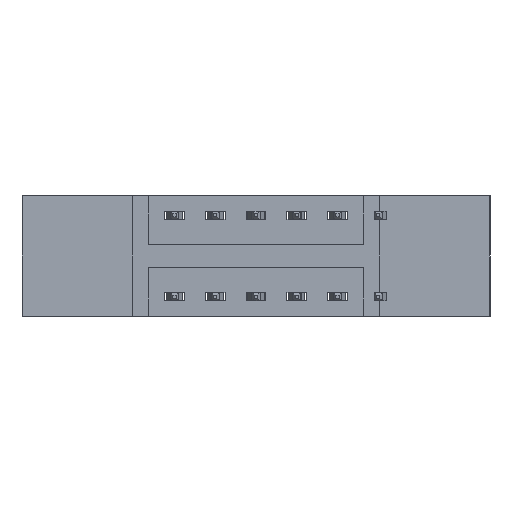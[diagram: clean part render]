
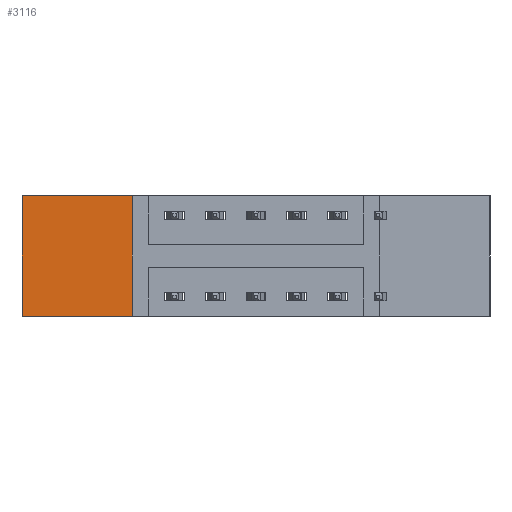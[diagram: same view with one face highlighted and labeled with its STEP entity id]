
A CAD part, front view. The second image highlights one B-rep face of the part: STEP entity #3116.
In plain terms, the highlighted planar face has unit normal (0, -1, 0).
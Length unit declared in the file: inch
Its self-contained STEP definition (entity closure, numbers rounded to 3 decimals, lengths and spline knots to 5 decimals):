
#100 = CARTESIAN_POINT ( 'NONE',  ( 0., 0.17, -0.37 ) ) ;
#230 = DIRECTION ( 'NONE',  ( 0., 0., 1. ) ) ;
#784 = DIRECTION ( 'NONE',  ( 1., 0., 0. ) ) ;
#1079 = EDGE_CURVE ( 'NONE', #4943, #7428, #5833, .T. ) ;
#1197 = CARTESIAN_POINT ( 'NONE',  ( 0.3375, 0.17, -0.37 ) ) ;
#1203 = CARTESIAN_POINT ( 'NONE',  ( 0.3375, 0.17, 0. ) ) ;
#1258 = CARTESIAN_POINT ( 'NONE',  ( 0., 0.17, 0. ) ) ;
#1836 = EDGE_CURVE ( 'NONE', #3618, #4943, #2764, .T. ) ;
#1899 = DIRECTION ( 'NONE',  ( -1., 0., 0. ) ) ;
#2666 = AXIS2_PLACEMENT_3D ( 'NONE', #4373, #3694, #6317 ) ;
#2764 = LINE ( 'NONE', #8026, #3585 ) ;
#2996 = FACE_OUTER_BOUND ( 'NONE', #7857, .T. ) ;
#3029 = ORIENTED_EDGE ( 'NONE', *, *, #1079, .T. ) ;
#3116 = ADVANCED_FACE ( 'NONE', ( #2996 ), #8420, .T. ) ;
#3242 = VECTOR ( 'NONE', #1899, 39.37008 ) ;
#3372 = LINE ( 'NONE', #4587, #5441 ) ;
#3415 = DIRECTION ( 'NONE',  ( 0., 0., -1. ) ) ;
#3585 = VECTOR ( 'NONE', #230, 39.37008 ) ;
#3618 = VERTEX_POINT ( 'NONE', #1197 ) ;
#3694 = DIRECTION ( 'NONE',  ( 0., -1., 0. ) ) ;
#4373 = CARTESIAN_POINT ( 'NONE',  ( 0., 0.17, -0.37 ) ) ;
#4587 = CARTESIAN_POINT ( 'NONE',  ( 0., 0.17, 0. ) ) ;
#4729 = EDGE_CURVE ( 'NONE', #7428, #5667, #3372, .T. ) ;
#4943 = VERTEX_POINT ( 'NONE', #1203 ) ;
#5441 = VECTOR ( 'NONE', #3415, 39.37008 ) ;
#5667 = VERTEX_POINT ( 'NONE', #6264 ) ;
#5815 = ORIENTED_EDGE ( 'NONE', *, *, #7746, .T. ) ;
#5833 = LINE ( 'NONE', #1258, #3242 ) ;
#5959 = LINE ( 'NONE', #100, #6807 ) ;
#5965 = ORIENTED_EDGE ( 'NONE', *, *, #1836, .T. ) ;
#6264 = CARTESIAN_POINT ( 'NONE',  ( 0., 0.17, -0.37 ) ) ;
#6294 = ORIENTED_EDGE ( 'NONE', *, *, #4729, .T. ) ;
#6317 = DIRECTION ( 'NONE',  ( 0., 0., -1. ) ) ;
#6807 = VECTOR ( 'NONE', #784, 39.37008 ) ;
#7428 = VERTEX_POINT ( 'NONE', #7589 ) ;
#7589 = CARTESIAN_POINT ( 'NONE',  ( 0., 0.17, 0. ) ) ;
#7746 = EDGE_CURVE ( 'NONE', #5667, #3618, #5959, .T. ) ;
#7857 = EDGE_LOOP ( 'NONE', ( #6294, #5815, #5965, #3029 ) ) ;
#8026 = CARTESIAN_POINT ( 'NONE',  ( 0.3375, 0.17, 0. ) ) ;
#8420 = PLANE ( 'NONE',  #2666 ) ;
